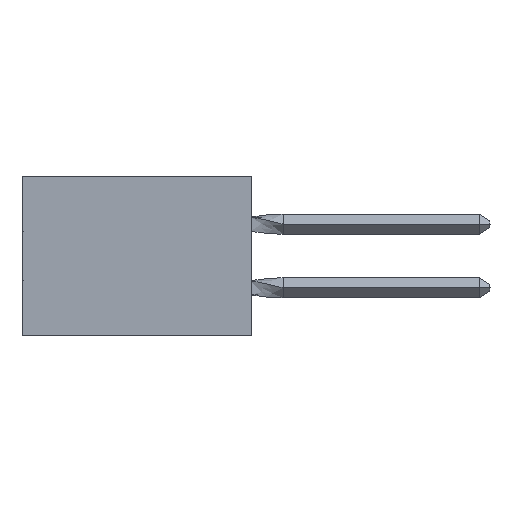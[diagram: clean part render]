
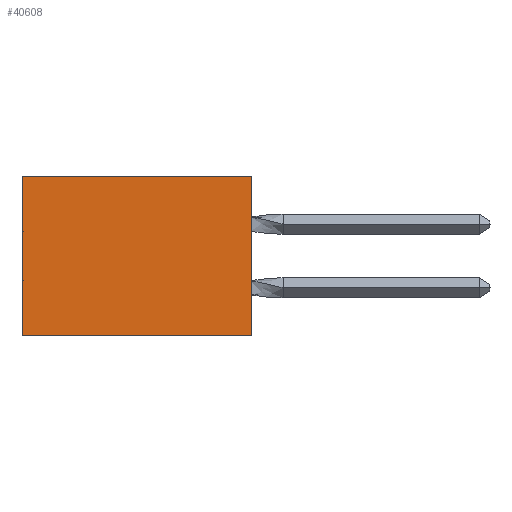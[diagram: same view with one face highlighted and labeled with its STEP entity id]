
A CAD part, left-side view. The second image highlights one B-rep face of the part: STEP entity #40608.
In plain terms, the highlighted planar face has unit normal (-1, 0, 0).
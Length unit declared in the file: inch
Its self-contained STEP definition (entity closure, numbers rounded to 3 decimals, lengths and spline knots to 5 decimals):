
#2842 = VERTEX_POINT ( 'NONE', #11702 ) ;
#3325 = VERTEX_POINT ( 'NONE', #30834 ) ;
#5909 = CARTESIAN_POINT ( 'NONE',  ( 0.305, 0., 0. ) ) ;
#7194 = DIRECTION ( 'NONE',  ( 0., 1., 0. ) ) ;
#9747 = DIRECTION ( 'NONE',  ( 0., 0., -1. ) ) ;
#10177 = PLANE ( 'NONE',  #30259 ) ;
#10420 = VECTOR ( 'NONE', #21154, 39.37008 ) ;
#10421 = CARTESIAN_POINT ( 'NONE',  ( 0.305, 0., -0.5 ) ) ;
#10825 = LINE ( 'NONE', #18063, #38121 ) ;
#11402 = CARTESIAN_POINT ( 'NONE',  ( 0.305, 0.72, -0.5 ) ) ;
#11702 = CARTESIAN_POINT ( 'NONE',  ( 0.305, 0., -0.5 ) ) ;
#13505 = DIRECTION ( 'NONE',  ( 0., 1., 0. ) ) ;
#18063 = CARTESIAN_POINT ( 'NONE',  ( 0.305, 0., -0.5 ) ) ;
#18548 = EDGE_CURVE ( 'NONE', #28163, #34696, #40335, .T. ) ;
#19259 = EDGE_CURVE ( 'NONE', #2842, #34696, #10825, .T. ) ;
#20447 = ORIENTED_EDGE ( 'NONE', *, *, #18548, .T. ) ;
#20759 = DIRECTION ( 'NONE',  ( 1., 0., 0. ) ) ;
#20913 = CARTESIAN_POINT ( 'NONE',  ( 0.305, 0., -0.5 ) ) ;
#21075 = DIRECTION ( 'NONE',  ( 0., 0., -1. ) ) ;
#21154 = DIRECTION ( 'NONE',  ( 0., 0., -1. ) ) ;
#21410 = VECTOR ( 'NONE', #9747, 39.37008 ) ;
#22620 = CARTESIAN_POINT ( 'NONE',  ( 0.305, 0.72, 0. ) ) ;
#24038 = CARTESIAN_POINT ( 'NONE',  ( 0.305, 0.72, -0.5 ) ) ;
#25504 = ORIENTED_EDGE ( 'NONE', *, *, #29574, .T. ) ;
#28163 = VERTEX_POINT ( 'NONE', #22620 ) ;
#29574 = EDGE_CURVE ( 'NONE', #3325, #28163, #32440, .T. ) ;
#30259 = AXIS2_PLACEMENT_3D ( 'NONE', #20913, #20759, #21075 ) ;
#30834 = CARTESIAN_POINT ( 'NONE',  ( 0.305, 0., 0. ) ) ;
#32440 = LINE ( 'NONE', #5909, #44188 ) ;
#32465 = FACE_OUTER_BOUND ( 'NONE', #36494, .T. ) ;
#34696 = VERTEX_POINT ( 'NONE', #11402 ) ;
#36494 = EDGE_LOOP ( 'NONE', ( #20447, #41468, #43168, #25504 ) ) ;
#38121 = VECTOR ( 'NONE', #7194, 39.37008 ) ;
#38673 = EDGE_CURVE ( 'NONE', #3325, #2842, #42188, .T. ) ;
#40335 = LINE ( 'NONE', #24038, #21410 ) ;
#40608 = ADVANCED_FACE ( 'NONE', ( #32465 ), #10177, .F. ) ;
#41468 = ORIENTED_EDGE ( 'NONE', *, *, #19259, .F. ) ;
#42188 = LINE ( 'NONE', #10421, #10420 ) ;
#43168 = ORIENTED_EDGE ( 'NONE', *, *, #38673, .F. ) ;
#44188 = VECTOR ( 'NONE', #13505, 39.37008 ) ;
